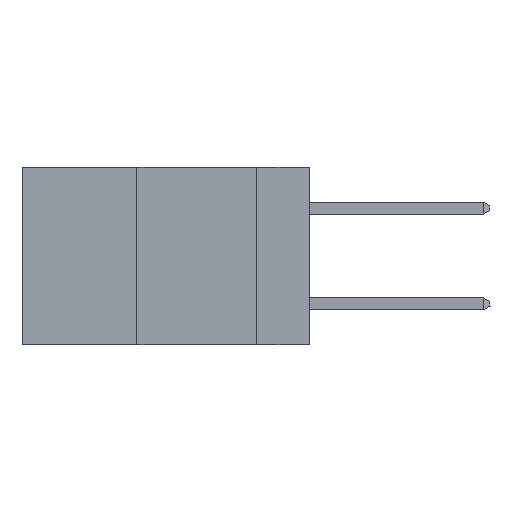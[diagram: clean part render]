
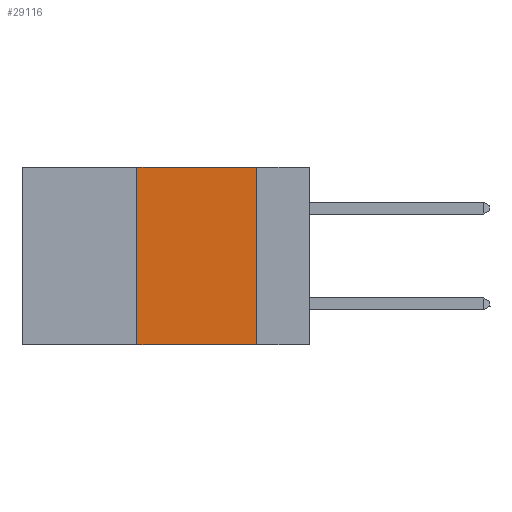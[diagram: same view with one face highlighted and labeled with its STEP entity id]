
A CAD part, left-side view. The second image highlights one B-rep face of the part: STEP entity #29116.
In plain terms, the highlighted planar face has unit normal (-1, 0, 0).
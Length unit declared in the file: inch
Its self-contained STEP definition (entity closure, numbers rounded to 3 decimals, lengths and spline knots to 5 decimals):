
#1422 = FACE_OUTER_BOUND ( 'NONE', #23381, .T. ) ;
#5245 = VERTEX_POINT ( 'NONE', #9132 ) ;
#9132 = CARTESIAN_POINT ( 'NONE',  ( 0., 0.11, -0.37 ) ) ;
#9757 = ORIENTED_EDGE ( 'NONE', *, *, #25916, .F. ) ;
#10436 = CARTESIAN_POINT ( 'NONE',  ( 0., 0.6, 0. ) ) ;
#10938 = EDGE_CURVE ( 'NONE', #37469, #5245, #30584, .T. ) ;
#11527 = CARTESIAN_POINT ( 'NONE',  ( 0., 0.6, 0. ) ) ;
#11854 = CARTESIAN_POINT ( 'NONE',  ( 0., 0.11, 0. ) ) ;
#11994 = ORIENTED_EDGE ( 'NONE', *, *, #10938, .T. ) ;
#12003 = DIRECTION ( 'NONE',  ( 0., 0., -1. ) ) ;
#15933 = DIRECTION ( 'NONE',  ( 0., -1., 0. ) ) ;
#17254 = DIRECTION ( 'NONE',  ( 0., -1., 0. ) ) ;
#18735 = LINE ( 'NONE', #11854, #22543 ) ;
#19741 = VECTOR ( 'NONE', #15933, 39.37008 ) ;
#19959 = ORIENTED_EDGE ( 'NONE', *, *, #37806, .F. ) ;
#21617 = CARTESIAN_POINT ( 'NONE',  ( 0., 0.11, 0. ) ) ;
#21680 = VECTOR ( 'NONE', #37481, 39.37008 ) ;
#22156 = DIRECTION ( 'NONE',  ( 1., 0., 0. ) ) ;
#22316 = DIRECTION ( 'NONE',  ( 0., 0., -1. ) ) ;
#22543 = VECTOR ( 'NONE', #12003, 39.37008 ) ;
#22664 = EDGE_CURVE ( 'NONE', #37469, #29558, #39523, .T. ) ;
#23381 = EDGE_LOOP ( 'NONE', ( #9757, #19959, #39662, #11994 ) ) ;
#24118 = CARTESIAN_POINT ( 'NONE',  ( 0., 0.36, 0. ) ) ;
#25160 = LINE ( 'NONE', #10436, #38615 ) ;
#25916 = EDGE_CURVE ( 'NONE', #28373, #5245, #18735, .T. ) ;
#27234 = CARTESIAN_POINT ( 'NONE',  ( 0., 0.36, 0. ) ) ;
#28373 = VERTEX_POINT ( 'NONE', #21617 ) ;
#29116 = ADVANCED_FACE ( 'NONE', ( #1422 ), #32309, .F. ) ;
#29558 = VERTEX_POINT ( 'NONE', #24118 ) ;
#30584 = LINE ( 'NONE', #40771, #19741 ) ;
#31662 = AXIS2_PLACEMENT_3D ( 'NONE', #11527, #22156, #22316 ) ;
#32309 = PLANE ( 'NONE',  #31662 ) ;
#32910 = CARTESIAN_POINT ( 'NONE',  ( 0., 0.36, -0.37 ) ) ;
#37469 = VERTEX_POINT ( 'NONE', #32910 ) ;
#37481 = DIRECTION ( 'NONE',  ( 0., 0., 1. ) ) ;
#37806 = EDGE_CURVE ( 'NONE', #29558, #28373, #25160, .T. ) ;
#38615 = VECTOR ( 'NONE', #17254, 39.37008 ) ;
#39523 = LINE ( 'NONE', #27234, #21680 ) ;
#39662 = ORIENTED_EDGE ( 'NONE', *, *, #22664, .F. ) ;
#40771 = CARTESIAN_POINT ( 'NONE',  ( 0., 0.6, -0.37 ) ) ;
